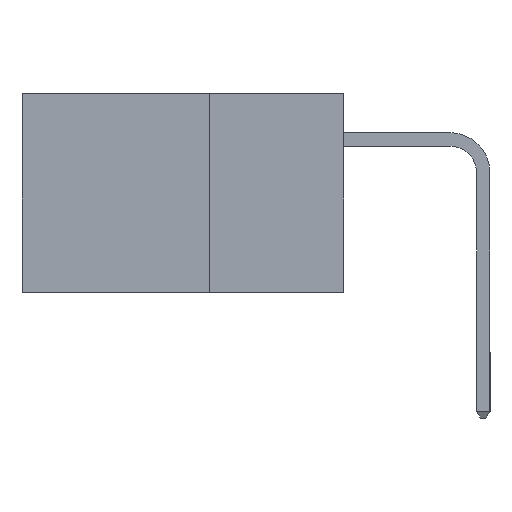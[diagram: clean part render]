
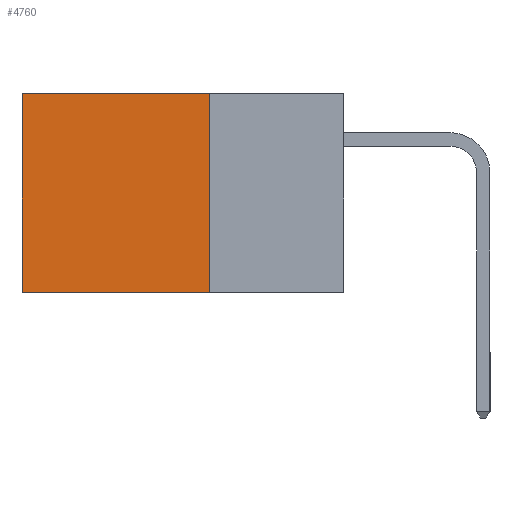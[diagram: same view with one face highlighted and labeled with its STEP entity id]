
A CAD part, left-side view. The second image highlights one B-rep face of the part: STEP entity #4760.
In plain terms, the highlighted planar face has unit normal (-1, 0, 0).
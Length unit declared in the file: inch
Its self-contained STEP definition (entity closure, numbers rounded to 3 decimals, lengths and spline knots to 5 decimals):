
#282 = LINE ( 'NONE', #4404, #5739 ) ;
#432 = EDGE_CURVE ( 'NONE', #8675, #3838, #7147, .T. ) ;
#791 = PLANE ( 'NONE',  #2169 ) ;
#824 = EDGE_CURVE ( 'NONE', #5315, #8675, #6751, .T. ) ;
#831 = VERTEX_POINT ( 'NONE', #4593 ) ;
#859 = DIRECTION ( 'NONE',  ( 0., 0., -1. ) ) ;
#1240 = CARTESIAN_POINT ( 'NONE',  ( 0.298, 0.6, 0. ) ) ;
#2079 = FACE_OUTER_BOUND ( 'NONE', #6753, .T. ) ;
#2169 = AXIS2_PLACEMENT_3D ( 'NONE', #4910, #3996, #859 ) ;
#2355 = VECTOR ( 'NONE', #5096, 39.37008 ) ;
#2574 = VECTOR ( 'NONE', #7921, 39.37008 ) ;
#2830 = CARTESIAN_POINT ( 'NONE',  ( 0.298, 0.25, 0. ) ) ;
#2837 = CARTESIAN_POINT ( 'NONE',  ( 0.298, 0.6, 0. ) ) ;
#3838 = VERTEX_POINT ( 'NONE', #6992 ) ;
#3996 = DIRECTION ( 'NONE',  ( 1., 0., 0. ) ) ;
#4404 = CARTESIAN_POINT ( 'NONE',  ( 0.298, 0.25, -0.37 ) ) ;
#4593 = CARTESIAN_POINT ( 'NONE',  ( 0.298, 0.25, -0.37 ) ) ;
#4760 = ADVANCED_FACE ( 'NONE', ( #2079 ), #791, .F. ) ;
#4910 = CARTESIAN_POINT ( 'NONE',  ( 0.298, 0.25, 0. ) ) ;
#5096 = DIRECTION ( 'NONE',  ( 0., 0., -1. ) ) ;
#5141 = DIRECTION ( 'NONE',  ( 0., 1., 0. ) ) ;
#5315 = VERTEX_POINT ( 'NONE', #7744 ) ;
#5428 = DIRECTION ( 'NONE',  ( 0., 1., 0. ) ) ;
#5655 = EDGE_CURVE ( 'NONE', #5315, #831, #6375, .T. ) ;
#5739 = VECTOR ( 'NONE', #5141, 39.37008 ) ;
#6375 = LINE ( 'NONE', #10227, #2574 ) ;
#6751 = LINE ( 'NONE', #2830, #9155 ) ;
#6753 = EDGE_LOOP ( 'NONE', ( #9449, #7057, #8002, #8052 ) ) ;
#6992 = CARTESIAN_POINT ( 'NONE',  ( 0.298, 0.6, -0.37 ) ) ;
#7057 = ORIENTED_EDGE ( 'NONE', *, *, #10007, .F. ) ;
#7147 = LINE ( 'NONE', #2837, #2355 ) ;
#7744 = CARTESIAN_POINT ( 'NONE',  ( 0.298, 0.25, 0. ) ) ;
#7921 = DIRECTION ( 'NONE',  ( 0., 0., -1. ) ) ;
#8002 = ORIENTED_EDGE ( 'NONE', *, *, #5655, .F. ) ;
#8052 = ORIENTED_EDGE ( 'NONE', *, *, #824, .T. ) ;
#8675 = VERTEX_POINT ( 'NONE', #1240 ) ;
#9155 = VECTOR ( 'NONE', #5428, 39.37008 ) ;
#9449 = ORIENTED_EDGE ( 'NONE', *, *, #432, .T. ) ;
#10007 = EDGE_CURVE ( 'NONE', #831, #3838, #282, .T. ) ;
#10227 = CARTESIAN_POINT ( 'NONE',  ( 0.298, 0.25, 0. ) ) ;
